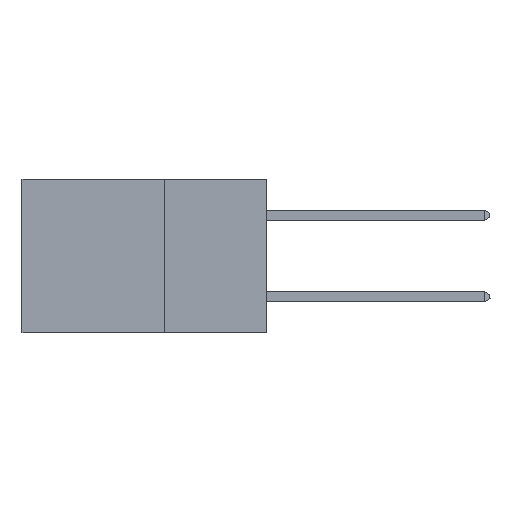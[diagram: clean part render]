
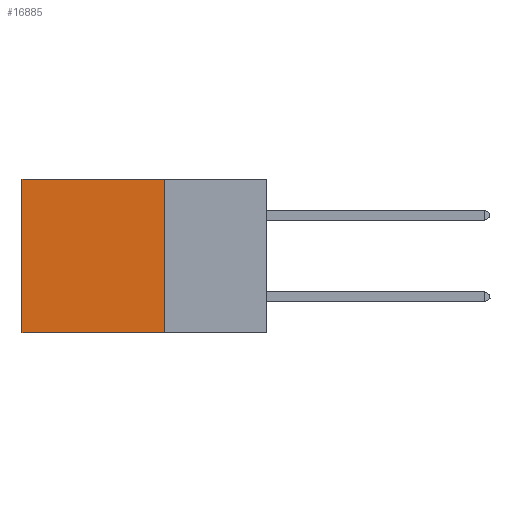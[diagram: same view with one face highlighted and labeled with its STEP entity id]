
A CAD part, left-side view. The second image highlights one B-rep face of the part: STEP entity #16885.
In plain terms, the highlighted planar face has unit normal (-1, 0, 0).
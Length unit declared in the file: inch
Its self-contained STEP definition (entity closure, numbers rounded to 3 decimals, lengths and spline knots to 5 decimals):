
#104 = FACE_OUTER_BOUND ( 'NONE', #8280, .T. ) ;
#544 = DIRECTION ( 'NONE',  ( 1., 0., 0. ) ) ;
#879 = VECTOR ( 'NONE', #21869, 39.37008 ) ;
#1539 = DIRECTION ( 'NONE',  ( 0., 1., 0. ) ) ;
#2197 = CARTESIAN_POINT ( 'NONE',  ( 0.2875, 0.6, -0.375 ) ) ;
#3384 = VERTEX_POINT ( 'NONE', #21935 ) ;
#3997 = DIRECTION ( 'NONE',  ( 0., 0., -1. ) ) ;
#5653 = LINE ( 'NONE', #5918, #879 ) ;
#5918 = CARTESIAN_POINT ( 'NONE',  ( 0.2875, 0.25, -0.375 ) ) ;
#6003 = CARTESIAN_POINT ( 'NONE',  ( 0.2875, 0.25, -0.375 ) ) ;
#8280 = EDGE_LOOP ( 'NONE', ( #12952, #16335, #10262, #11738 ) ) ;
#8695 = LINE ( 'NONE', #20856, #22369 ) ;
#8765 = CARTESIAN_POINT ( 'NONE',  ( 0.2875, 0.25, 0. ) ) ;
#10262 = ORIENTED_EDGE ( 'NONE', *, *, #17452, .F. ) ;
#10945 = AXIS2_PLACEMENT_3D ( 'NONE', #16678, #544, #11439 ) ;
#11439 = DIRECTION ( 'NONE',  ( 0., 0., -1. ) ) ;
#11738 = ORIENTED_EDGE ( 'NONE', *, *, #15022, .T. ) ;
#11978 = DIRECTION ( 'NONE',  ( 0., 1., 0. ) ) ;
#12042 = EDGE_CURVE ( 'NONE', #23041, #18426, #8695, .T. ) ;
#12952 = ORIENTED_EDGE ( 'NONE', *, *, #16168, .T. ) ;
#13902 = CARTESIAN_POINT ( 'NONE',  ( 0.2875, 0.25, 0. ) ) ;
#14420 = VECTOR ( 'NONE', #3997, 39.37008 ) ;
#15022 = EDGE_CURVE ( 'NONE', #19525, #3384, #19481, .T. ) ;
#15047 = PLANE ( 'NONE',  #10945 ) ;
#16168 = EDGE_CURVE ( 'NONE', #3384, #18426, #17763, .T. ) ;
#16335 = ORIENTED_EDGE ( 'NONE', *, *, #12042, .F. ) ;
#16478 = CARTESIAN_POINT ( 'NONE',  ( 0.2875, 0.6, -0.375 ) ) ;
#16678 = CARTESIAN_POINT ( 'NONE',  ( 0.2875, 0.25, -0.375 ) ) ;
#16885 = ADVANCED_FACE ( 'NONE', ( #104 ), #15047, .F. ) ;
#17452 = EDGE_CURVE ( 'NONE', #19525, #23041, #5653, .T. ) ;
#17763 = LINE ( 'NONE', #16478, #14420 ) ;
#18426 = VERTEX_POINT ( 'NONE', #2197 ) ;
#19481 = LINE ( 'NONE', #8765, #20567 ) ;
#19525 = VERTEX_POINT ( 'NONE', #13902 ) ;
#20567 = VECTOR ( 'NONE', #1539, 39.37008 ) ;
#20856 = CARTESIAN_POINT ( 'NONE',  ( 0.2875, 0.25, -0.375 ) ) ;
#21869 = DIRECTION ( 'NONE',  ( 0., 0., -1. ) ) ;
#21935 = CARTESIAN_POINT ( 'NONE',  ( 0.2875, 0.6, 0. ) ) ;
#22369 = VECTOR ( 'NONE', #11978, 39.37008 ) ;
#23041 = VERTEX_POINT ( 'NONE', #6003 ) ;
